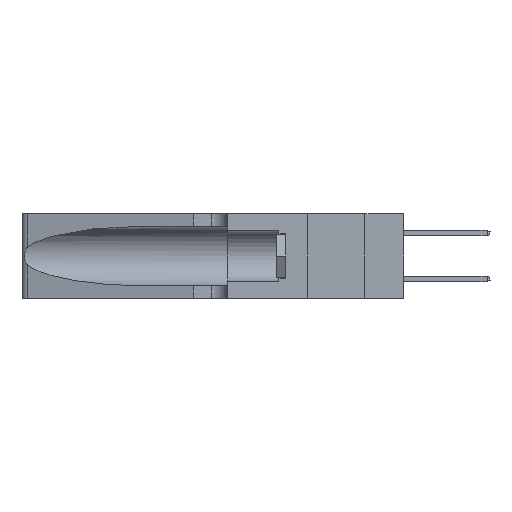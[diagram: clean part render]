
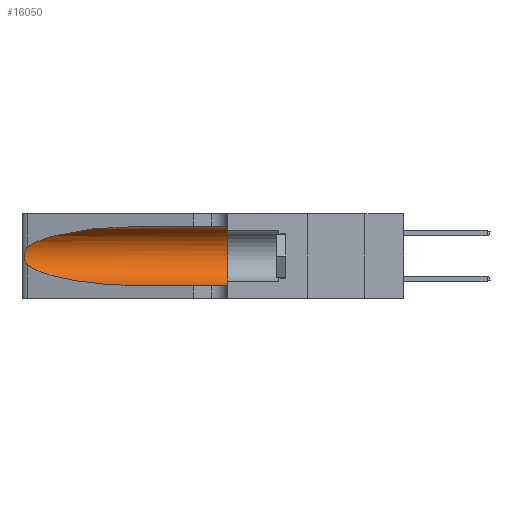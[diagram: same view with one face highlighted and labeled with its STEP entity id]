
A CAD part, left-side view. The second image highlights one B-rep face of the part: STEP entity #16050.
In plain terms, the highlighted cylindrical face has radius 3.308 mm (diameter 6.617 mm), a partial arc.
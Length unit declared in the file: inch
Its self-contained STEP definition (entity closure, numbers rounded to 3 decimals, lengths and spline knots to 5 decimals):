
#297 = CARTESIAN_POINT ( 'NONE',  ( 0.1305, 0.72297, 0.31525 ) ) ;
#751 = CARTESIAN_POINT ( 'NONE',  ( 0.18966, 0.96281, 0.05475 ) ) ;
#837 = CARTESIAN_POINT ( 'NONE',  ( 0.26018, 1.23835, 0.19895 ) ) ;
#1253 = CARTESIAN_POINT ( 'NONE',  ( 0.1305, 0.72297, 0.31525 ) ) ;
#1774 = CARTESIAN_POINT ( 'NONE',  ( 0.25487, 1.22718, 0.22369 ) ) ;
#2697 = CYLINDRICAL_SURFACE ( 'NONE', #14648, 0.13025 ) ;
#2753 = VERTEX_POINT ( 'NONE', #1774 ) ;
#2973 = ORIENTED_EDGE ( 'NONE', *, *, #15677, .F. ) ;
#3041 = CARTESIAN_POINT ( 'NONE',  ( 0.26075, 1.23896, 0.178 ) ) ;
#3362 = EDGE_CURVE ( 'NONE', #5437, #26775, #22119, .T. ) ;
#3859 = VERTEX_POINT ( 'NONE', #18823 ) ;
#3863 = CARTESIAN_POINT ( 'NONE',  ( 0.1305, 0.35, 0.185 ) ) ;
#4359 = VECTOR ( 'NONE', #21941, 39.37008 ) ;
#4655 = ORIENTED_EDGE ( 'NONE', *, *, #20096, .T. ) ;
#4658 = CARTESIAN_POINT ( 'NONE',  ( 0.25487, 1.22718, 0.22369 ) ) ;
#5110 = CARTESIAN_POINT ( 'NONE',  ( 0.25555, 1.22994, 0.2215 ) ) ;
#5198 = CARTESIAN_POINT ( 'NONE',  ( 0.25856, 1.23593, 0.16098 ) ) ;
#5242 = EDGE_LOOP ( 'NONE', ( #4655, #10845, #21730, #12769, #2973, #14033 ) ) ;
#5437 = VERTEX_POINT ( 'NONE', #1253 ) ;
#5725 = VECTOR ( 'NONE', #11384, 39.37008 ) ;
#5986 = DIRECTION ( 'NONE',  ( 0., 0., 1. ) ) ;
#6777 = B_SPLINE_CURVE_WITH_KNOTS ( 'NONE', 3,
 ( #21476, #5110, #11359, #25641, #13407, #837, #15445, #3041, #17464, #5198, #19537, #7295, #22027, #9775 ),
 .UNSPECIFIED., .F., .F.,
 ( 4, 2, 2, 2, 2, 2, 4 ),
 ( 0., 0.00027, 0.00053, 0.00107, 0.0016, 0.00187, 0.00214 ),
 .UNSPECIFIED. ) ;
#7295 = CARTESIAN_POINT ( 'NONE',  ( 0.25639, 1.23186, 0.15144 ) ) ;
#8142 = VERTEX_POINT ( 'NONE', #22974 ) ;
#8315 = AXIS2_PLACEMENT_3D ( 'NONE', #3863, #18250, #5986 ) ;
#9160 = CARTESIAN_POINT ( 'NONE',  ( 0.1305, 1.61858, 0.185 ) ) ;
#9689 = CARTESIAN_POINT ( 'NONE',  ( 0.1305, 1.61858, 0.05475 ) ) ;
#9705 = VERTEX_POINT ( 'NONE', #25766 ) ;
#9775 = CARTESIAN_POINT ( 'NONE',  ( 0.25487, 1.22718, 0.14631 ) ) ;
#10845 = ORIENTED_EDGE ( 'NONE', *, *, #18360, .T. ) ;
#11359 = CARTESIAN_POINT ( 'NONE',  ( 0.25639, 1.23184, 0.21858 ) ) ;
#11384 = DIRECTION ( 'NONE',  ( 0., -1., 0. ) ) ;
#12769 = ORIENTED_EDGE ( 'NONE', *, *, #23586, .T. ) ;
#13407 = CARTESIAN_POINT ( 'NONE',  ( 0.25854, 1.2359, 0.20912 ) ) ;
#14033 = ORIENTED_EDGE ( 'NONE', *, *, #3362, .F. ) ;
#14111 = EDGE_CURVE ( 'NONE', #3859, #9705, #25818, .T. ) ;
#14648 = AXIS2_PLACEMENT_3D ( 'NONE', #9160, #19290, #23468 ) ;
#14798 = CARTESIAN_POINT ( 'NONE',  ( 0.1305, 0.35, 0.31525 ) ) ;
#14924 = CARTESIAN_POINT ( 'NONE',  ( 0.18966, 0.96281, 0.31525 ) ) ;
#15306 = LINE ( 'NONE', #9689, #4359 ) ;
#15362 = CARTESIAN_POINT ( 'NONE',  ( 0.1305, 0.72297, 0.05475 ) ) ;
#15380 = CARTESIAN_POINT ( 'NONE',  ( 0.1305, 1.61858, 0.31525 ) ) ;
#15445 = CARTESIAN_POINT ( 'NONE',  ( 0.26075, 1.23896, 0.19203 ) ) ;
#15677 = EDGE_CURVE ( 'NONE', #26775, #8142, #17926, .T. ) ;
#16050 = ADVANCED_FACE ( 'NONE', ( #19178 ), #2697, .F. ) ;
#16936 = CARTESIAN_POINT ( 'NONE',  ( 0.2373, 1.15595, 0.28018 ) ) ;
#17290 = CARTESIAN_POINT ( 'NONE',  ( 0.2373, 1.15595, 0.08982 ) ) ;
#17464 = CARTESIAN_POINT ( 'NONE',  ( 0.26017, 1.23833, 0.17102 ) ) ;
#17926 = CIRCLE ( 'NONE', #8315, 0.13025 ) ;
#18250 = DIRECTION ( 'NONE',  ( 0., 1., 0. ) ) ;
#18360 = EDGE_CURVE ( 'NONE', #2753, #3859, #6777, .T. ) ;
#18823 = CARTESIAN_POINT ( 'NONE',  ( 0.25487, 1.22718, 0.14631 ) ) ;
#19178 = FACE_OUTER_BOUND ( 'NONE', #5242, .T. ) ;
#19290 = DIRECTION ( 'NONE',  ( 0., -1., 0. ) ) ;
#19537 = CARTESIAN_POINT ( 'NONE',  ( 0.25789, 1.23486, 0.15765 ) ) ;
#20096 = EDGE_CURVE ( 'NONE', #5437, #2753, #23890, .T. ) ;
#21476 = CARTESIAN_POINT ( 'NONE',  ( 0.25487, 1.22718, 0.22369 ) ) ;
#21730 = ORIENTED_EDGE ( 'NONE', *, *, #14111, .T. ) ;
#21941 = DIRECTION ( 'NONE',  ( 0., -1., 0. ) ) ;
#22027 = CARTESIAN_POINT ( 'NONE',  ( 0.25555, 1.22993, 0.14849 ) ) ;
#22119 = LINE ( 'NONE', #15380, #5725 ) ;
#22974 = CARTESIAN_POINT ( 'NONE',  ( 0.1305, 0.35, 0.05475 ) ) ;
#23468 = DIRECTION ( 'NONE',  ( 0., 0., -1. ) ) ;
#23586 = EDGE_CURVE ( 'NONE', #9705, #8142, #15306, .T. ) ;
#23890 =( BOUNDED_CURVE ( )  B_SPLINE_CURVE ( 3, ( #297, #14924, #16936, #4658 ),
 .UNSPECIFIED., .F., .F. ) 
 B_SPLINE_CURVE_WITH_KNOTS ( ( 4, 4 ),
 ( 1.5708, 2.84003 ),
 .UNSPECIFIED. ) 
 CURVE ( )  GEOMETRIC_REPRESENTATION_ITEM ( )  RATIONAL_B_SPLINE_CURVE ( ( 1., 0.87, 0.87, 1. ) ) 
 REPRESENTATION_ITEM ( '' )  );
#25562 = CARTESIAN_POINT ( 'NONE',  ( 0.25487, 1.22718, 0.14631 ) ) ;
#25641 = CARTESIAN_POINT ( 'NONE',  ( 0.25787, 1.23484, 0.2124 ) ) ;
#25766 = CARTESIAN_POINT ( 'NONE',  ( 0.1305, 0.72297, 0.05475 ) ) ;
#25818 =( BOUNDED_CURVE ( )  B_SPLINE_CURVE ( 3, ( #25562, #17290, #751, #15362 ),
 .UNSPECIFIED., .F., .F. ) 
 B_SPLINE_CURVE_WITH_KNOTS ( ( 4, 4 ),
 ( 3.44316, 4.71239 ),
 .UNSPECIFIED. ) 
 CURVE ( )  GEOMETRIC_REPRESENTATION_ITEM ( )  RATIONAL_B_SPLINE_CURVE ( ( 1., 0.87, 0.87, 1. ) ) 
 REPRESENTATION_ITEM ( '' )  );
#26775 = VERTEX_POINT ( 'NONE', #14798 ) ;
